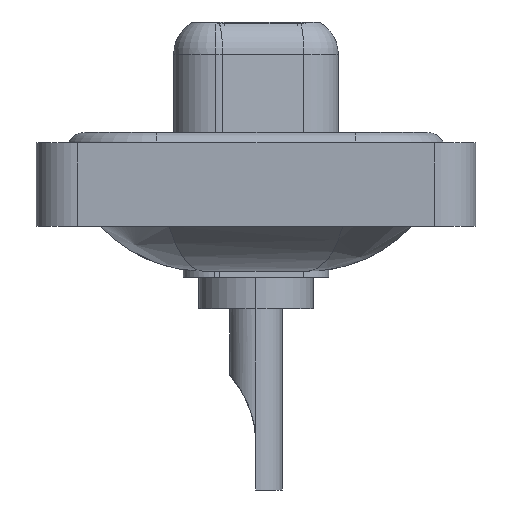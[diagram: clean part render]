
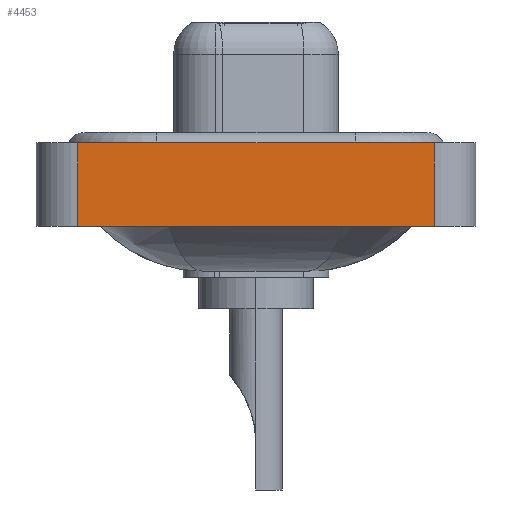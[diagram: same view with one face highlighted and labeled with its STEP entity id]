
A CAD part, left-side view. The second image highlights one B-rep face of the part: STEP entity #4453.
In plain terms, the highlighted planar face has unit normal (-1, 0, 0).
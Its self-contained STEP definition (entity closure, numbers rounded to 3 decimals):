
#408 = EDGE_LOOP ( 'NONE', ( #11588, #15551, #10937, #16958 ) ) ;
#876 = VECTOR ( 'NONE', #1494, 1000. ) ;
#1494 = DIRECTION ( 'NONE',  ( 0., 0., 1. ) ) ;
#2823 = CARTESIAN_POINT ( 'NONE',  ( -7.3, 8.55, -3.6 ) ) ;
#2911 = LINE ( 'NONE', #2823, #876 ) ;
#2995 = CARTESIAN_POINT ( 'NONE',  ( -7.3, -8.55, -3.6 ) ) ;
#4453 = ADVANCED_FACE ( 'NONE', ( #11836 ), #7625, .T. ) ;
#4887 = CARTESIAN_POINT ( 'NONE',  ( -7.3, -8.55, -3.6 ) ) ;
#5024 = CARTESIAN_POINT ( 'NONE',  ( -7.3, -8.55, -3.6 ) ) ;
#5164 = EDGE_CURVE ( 'NONE', #16349, #8244, #13040, .T. ) ;
#5370 = CARTESIAN_POINT ( 'NONE',  ( -7.3, -8.55, -3.6 ) ) ;
#7625 = PLANE ( 'NONE',  #9688 ) ;
#7845 = VECTOR ( 'NONE', #14282, 1000. ) ;
#8149 = VERTEX_POINT ( 'NONE', #14357 ) ;
#8244 = VERTEX_POINT ( 'NONE', #5370 ) ;
#9056 = DIRECTION ( 'NONE',  ( -1., 0., 0. ) ) ;
#9688 = AXIS2_PLACEMENT_3D ( 'NONE', #4887, #9056, #13257 ) ;
#10544 = EDGE_CURVE ( 'NONE', #16349, #11084, #2911, .T. ) ;
#10588 = EDGE_CURVE ( 'NONE', #8244, #8149, #15194, .T. ) ;
#10937 = ORIENTED_EDGE ( 'NONE', *, *, #10544, .F. ) ;
#11084 = VERTEX_POINT ( 'NONE', #16949 ) ;
#11588 = ORIENTED_EDGE ( 'NONE', *, *, #10588, .T. ) ;
#11836 = FACE_OUTER_BOUND ( 'NONE', #408, .T. ) ;
#11894 = LINE ( 'NONE', #13227, #12813 ) ;
#12155 = DIRECTION ( 'NONE',  ( 0., -1., 0. ) ) ;
#12708 = CARTESIAN_POINT ( 'NONE',  ( -7.3, 8.55, -3.6 ) ) ;
#12813 = VECTOR ( 'NONE', #12155, 1000. ) ;
#12824 = VECTOR ( 'NONE', #15278, 1000. ) ;
#13040 = LINE ( 'NONE', #5024, #7845 ) ;
#13227 = CARTESIAN_POINT ( 'NONE',  ( -7.3, -8.55, 0.4 ) ) ;
#13257 = DIRECTION ( 'NONE',  ( 0., 0., 1. ) ) ;
#14282 = DIRECTION ( 'NONE',  ( 0., -1., 0. ) ) ;
#14357 = CARTESIAN_POINT ( 'NONE',  ( -7.3, -8.55, 0.4 ) ) ;
#15194 = LINE ( 'NONE', #2995, #12824 ) ;
#15278 = DIRECTION ( 'NONE',  ( 0., 0., 1. ) ) ;
#15551 = ORIENTED_EDGE ( 'NONE', *, *, #15763, .F. ) ;
#15763 = EDGE_CURVE ( 'NONE', #11084, #8149, #11894, .T. ) ;
#16349 = VERTEX_POINT ( 'NONE', #12708 ) ;
#16949 = CARTESIAN_POINT ( 'NONE',  ( -7.3, 8.55, 0.4 ) ) ;
#16958 = ORIENTED_EDGE ( 'NONE', *, *, #5164, .T. ) ;
